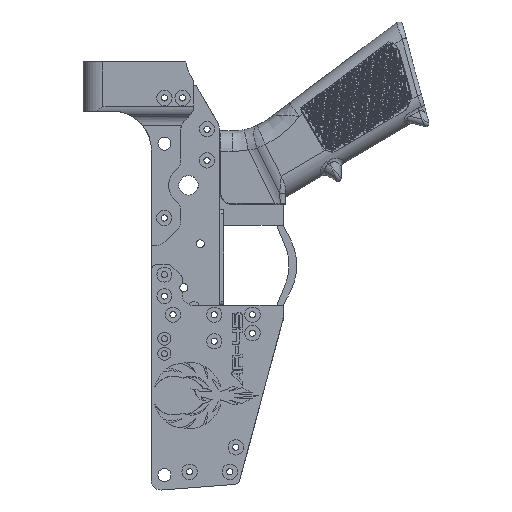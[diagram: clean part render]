
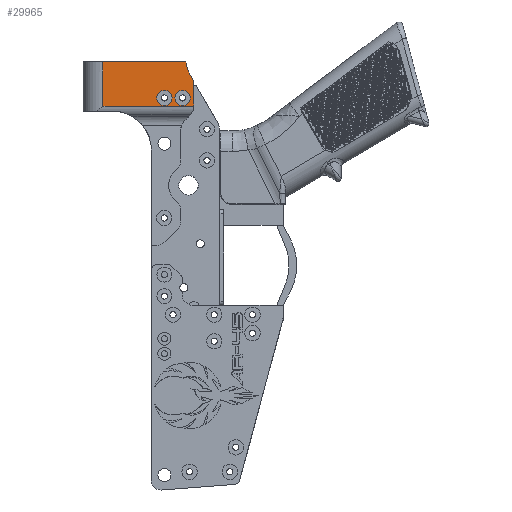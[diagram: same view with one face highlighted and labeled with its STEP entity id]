
A CAD part, left-side view. The second image highlights one B-rep face of the part: STEP entity #29965.
In plain terms, the highlighted planar face has unit normal (-1, 0, 0).
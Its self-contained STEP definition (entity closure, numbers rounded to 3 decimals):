
#11026 = DIRECTION ( 'NONE',  ( 0., 0., -1. ) ) ;
#12397 = CARTESIAN_POINT ( 'NONE',  ( -25., -36.779, 1.76 ) ) ;
#14503 = EDGE_CURVE ( 'NONE', #24015, #83521, #251121, .T. ) ;
#16048 = CARTESIAN_POINT ( 'NONE',  ( -25., -22.327, -2.6 ) ) ;
#21056 = CIRCLE ( 'NONE', #221813, 3.75 ) ;
#22726 = DIRECTION ( 'NONE',  ( -1., 0., 0. ) ) ;
#24015 = VERTEX_POINT ( 'NONE', #76271 ) ;
#24245 = CIRCLE ( 'NONE', #179036, 3.75 ) ;
#24653 = VECTOR ( 'NONE', #11026, 1000. ) ;
#25793 = DIRECTION ( 'NONE',  ( 0., 0.5, 0.866 ) ) ;
#26996 = ORIENTED_EDGE ( 'NONE', *, *, #63777, .F. ) ;
#27310 = EDGE_CURVE ( 'NONE', #213105, #122969, #56481, .T. ) ;
#28760 = DIRECTION ( 'NONE',  ( 1., 0., 0. ) ) ;
#29373 = ORIENTED_EDGE ( 'NONE', *, *, #14503, .F. ) ;
#29965 = ADVANCED_FACE ( 'NONE', ( #165396, #167948, #186282 ), #242693, .F. ) ;
#30819 = VECTOR ( 'NONE', #76086, 1000. ) ;
#31167 = DIRECTION ( 'NONE',  ( 0., 0., 1. ) ) ;
#31342 = DIRECTION ( 'NONE',  ( 0., 0., -1. ) ) ;
#31933 = LINE ( 'NONE', #172041, #24653 ) ;
#32435 = DIRECTION ( 'NONE',  ( -1., 0., 0. ) ) ;
#36619 = VERTEX_POINT ( 'NONE', #12397 ) ;
#37331 = AXIS2_PLACEMENT_3D ( 'NONE', #168872, #28760, #31342 ) ;
#40220 = CARTESIAN_POINT ( 'NONE',  ( -25., -32.853, 11.224 ) ) ;
#43349 = EDGE_LOOP ( 'NONE', ( #26996, #87649 ) ) ;
#44068 = EDGE_LOOP ( 'NONE', ( #94619, #140145, #114334, #88506, #234809, #208006 ) ) ;
#52701 = DIRECTION ( 'NONE',  ( 0., 0., 1. ) ) ;
#56481 = LINE ( 'NONE', #254153, #30819 ) ;
#63777 = EDGE_CURVE ( 'NONE', #64147, #68296, #127890, .T. ) ;
#64147 = VERTEX_POINT ( 'NONE', #192443 ) ;
#65866 = DIRECTION ( 'NONE',  ( 0., 0., -1. ) ) ;
#68296 = VERTEX_POINT ( 'NONE', #248838 ) ;
#70109 = VERTEX_POINT ( 'NONE', #148793 ) ;
#74090 = EDGE_CURVE ( 'NONE', #68296, #64147, #21056, .T. ) ;
#76086 = DIRECTION ( 'NONE',  ( 0., -1., 0. ) ) ;
#76271 = CARTESIAN_POINT ( 'NONE',  ( -25., -22.327, -10.1 ) ) ;
#77782 = DIRECTION ( 'NONE',  ( 0., 0., 1. ) ) ;
#83457 = LINE ( 'NONE', #203894, #161601 ) ;
#83521 = VERTEX_POINT ( 'NONE', #16048 ) ;
#87537 = VERTEX_POINT ( 'NONE', #40220 ) ;
#87649 = ORIENTED_EDGE ( 'NONE', *, *, #74090, .F. ) ;
#88506 = ORIENTED_EDGE ( 'NONE', *, *, #188447, .T. ) ;
#91851 = EDGE_CURVE ( 'NONE', #83521, #24015, #24245, .T. ) ;
#94619 = ORIENTED_EDGE ( 'NONE', *, *, #253380, .T. ) ;
#97861 = VECTOR ( 'NONE', #179524, 1000. ) ;
#100573 = DIRECTION ( 'NONE',  ( 0., 0., 1. ) ) ;
#105706 = LINE ( 'NONE', #244519, #170766 ) ;
#106452 = CARTESIAN_POINT ( 'NONE',  ( -25., -36.779, -288600.29 ) ) ;
#112507 = ORIENTED_EDGE ( 'NONE', *, *, #91851, .F. ) ;
#114334 = ORIENTED_EDGE ( 'NONE', *, *, #171484, .T. ) ;
#116801 = CARTESIAN_POINT ( 'NONE',  ( -25., -31.217, -6.35 ) ) ;
#118016 = CARTESIAN_POINT ( 'NONE',  ( -25., -36.779, 11.224 ) ) ;
#119920 = DIRECTION ( 'NONE',  ( 0., 0., 1. ) ) ;
#122969 = VERTEX_POINT ( 'NONE', #215954 ) ;
#127890 = CIRCLE ( 'NONE', #224175, 3.75 ) ;
#128642 = DIRECTION ( 'NONE',  ( 1., 0., 0. ) ) ;
#129492 = EDGE_CURVE ( 'NONE', #70109, #87537, #229637, .T. ) ;
#138291 = AXIS2_PLACEMENT_3D ( 'NONE', #176286, #232624, #119920 ) ;
#140145 = ORIENTED_EDGE ( 'NONE', *, *, #27310, .T. ) ;
#141904 = CARTESIAN_POINT ( 'NONE',  ( -25., -31.217, -6.35 ) ) ;
#148793 = CARTESIAN_POINT ( 'NONE',  ( -25., -34.789, 5.207 ) ) ;
#161601 = VECTOR ( 'NONE', #25793, 1000. ) ;
#163096 = CARTESIAN_POINT ( 'NONE',  ( -25., 7.678, 11.224 ) ) ;
#165396 = FACE_BOUND ( 'NONE', #43349, .T. ) ;
#167948 = FACE_BOUND ( 'NONE', #210924, .T. ) ;
#168872 = CARTESIAN_POINT ( 'NONE',  ( -25., -47.779, 12.707 ) ) ;
#169350 = AXIS2_PLACEMENT_3D ( 'NONE', #106452, #128642, #65866 ) ;
#170766 = VECTOR ( 'NONE', #100573, 1000. ) ;
#171484 = EDGE_CURVE ( 'NONE', #122969, #36619, #105706, .T. ) ;
#172041 = CARTESIAN_POINT ( 'NONE',  ( -25., 7.678, -12.776 ) ) ;
#176286 = CARTESIAN_POINT ( 'NONE',  ( -25., -22.327, -6.35 ) ) ;
#178250 = LINE ( 'NONE', #118016, #97861 ) ;
#179036 = AXIS2_PLACEMENT_3D ( 'NONE', #252400, #32435, #31167 ) ;
#179524 = DIRECTION ( 'NONE',  ( 0., 1., 0. ) ) ;
#185080 = EDGE_CURVE ( 'NONE', #87537, #211486, #178250, .T. ) ;
#186282 = FACE_OUTER_BOUND ( 'NONE', #44068, .T. ) ;
#188447 = EDGE_CURVE ( 'NONE', #36619, #70109, #83457, .T. ) ;
#192443 = CARTESIAN_POINT ( 'NONE',  ( -25., -31.217, -2.6 ) ) ;
#203894 = CARTESIAN_POINT ( 'NONE',  ( -25., -32.779, 8.688 ) ) ;
#208006 = ORIENTED_EDGE ( 'NONE', *, *, #185080, .T. ) ;
#210924 = EDGE_LOOP ( 'NONE', ( #112507, #29373 ) ) ;
#211132 = DIRECTION ( 'NONE',  ( -1., 0., 0. ) ) ;
#211486 = VERTEX_POINT ( 'NONE', #163096 ) ;
#213105 = VERTEX_POINT ( 'NONE', #216879 ) ;
#215954 = CARTESIAN_POINT ( 'NONE',  ( -25., -36.779, -10.291 ) ) ;
#216879 = CARTESIAN_POINT ( 'NONE',  ( -25., 7.678, -10.291 ) ) ;
#221813 = AXIS2_PLACEMENT_3D ( 'NONE', #141904, #22726, #77782 ) ;
#224175 = AXIS2_PLACEMENT_3D ( 'NONE', #116801, #211132, #52701 ) ;
#229637 = CIRCLE ( 'NONE', #37331, 15. ) ;
#232624 = DIRECTION ( 'NONE',  ( -1., 0., 0. ) ) ;
#234809 = ORIENTED_EDGE ( 'NONE', *, *, #129492, .T. ) ;
#242693 = PLANE ( 'NONE',  #169350 ) ;
#244519 = CARTESIAN_POINT ( 'NONE',  ( -25., -36.779, -288600.29 ) ) ;
#248838 = CARTESIAN_POINT ( 'NONE',  ( -25., -31.217, -10.1 ) ) ;
#251121 = CIRCLE ( 'NONE', #138291, 3.75 ) ;
#252400 = CARTESIAN_POINT ( 'NONE',  ( -25., -22.327, -6.35 ) ) ;
#253380 = EDGE_CURVE ( 'NONE', #211486, #213105, #31933, .T. ) ;
#254153 = CARTESIAN_POINT ( 'NONE',  ( -25., -36.779, -10.291 ) ) ;
